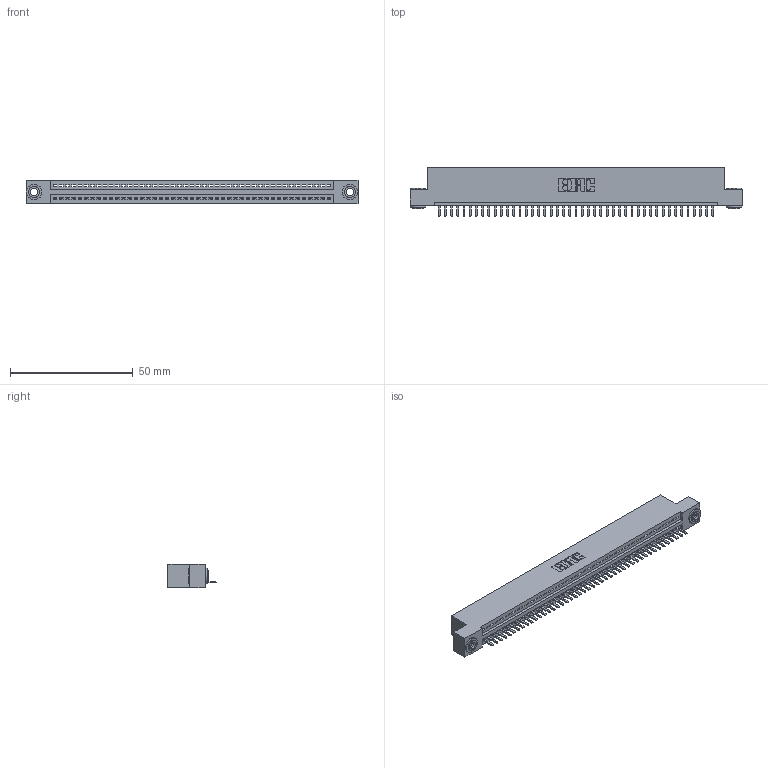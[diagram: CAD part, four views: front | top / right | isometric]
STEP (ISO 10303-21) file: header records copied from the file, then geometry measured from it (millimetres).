
FILE_DESCRIPTION (( 'STEP AP203' ), '1' );
FILE_NAME ('395-045-520-103.STEP', '2019-10-22T17:27:17', ( '' ), ( '' ), 'SwSTEP 2.0', 'SolidWorks 2016', '' );
FILE_SCHEMA (( 'CONFIG_CONTROL_DESIGN' ));
Length unit declared in the file: inch
Products named in the file (4): 345-250-002_345-250-002-102; 345 Part_Flush Mounting Lugs - 0.156 Dia-TH; 395-045-520-103; 345-292-001_345-293-120
Assembly tree (48 placements, depth 2):
  395-045-520-103
    345 Part_Flush Mounting Lugs - 0.156 Dia-TH
    345-292-001_345-293-120  x45
    345-250-002_345-250-002-102  x2
Bounding box: 135.51 x 19.68 x 9.4 mm (x, y, z)
Volume: 12785.3 mm3; surface area: 16822.3 mm2
Topology: 48 solids, 48 shells, 2954 faces, 8697 edges, 5674 vertices
Faces by surface type: plane 1980, cylinder 966, cone 8
Entity records: 34228 total; most frequent: CARTESIAN_POINT 5918, ORIENTED_EDGE 5878, DIRECTION 5183, EDGE_CURVE 2939, LINE 2599, VECTOR 2599, VERTEX_POINT 1954, AXIS2_PLACEMENT_3D 1292
